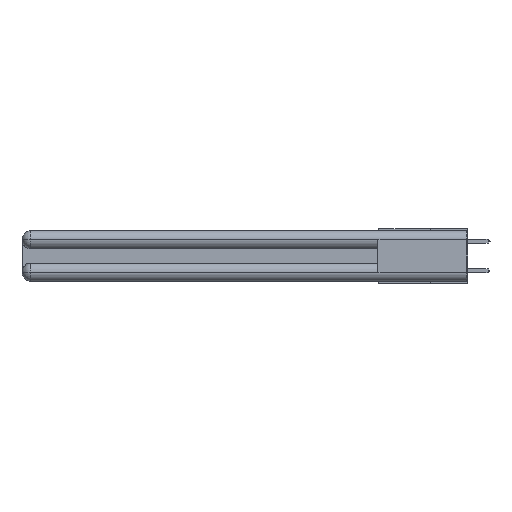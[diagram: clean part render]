
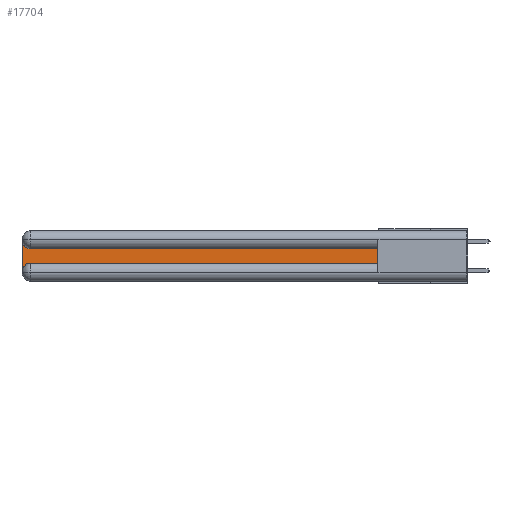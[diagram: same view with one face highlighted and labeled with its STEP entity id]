
A CAD part, left-side view. The second image highlights one B-rep face of the part: STEP entity #17704.
In plain terms, the highlighted planar face has unit normal (-1, 0, 0).
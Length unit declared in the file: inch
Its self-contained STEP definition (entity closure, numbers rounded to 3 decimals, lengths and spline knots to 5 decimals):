
#443 = DIRECTION ( 'NONE',  ( 1., 0., 0. ) ) ;
#962 = EDGE_CURVE ( 'NONE', #9273, #19125, #4611, .T. ) ;
#1816 = CARTESIAN_POINT ( 'NONE',  ( 0.075, 2.94, -0.2175 ) ) ;
#1875 = EDGE_CURVE ( 'NONE', #1937, #10689, #21821, .T. ) ;
#1937 = VERTEX_POINT ( 'NONE', #1816 ) ;
#2377 = VERTEX_POINT ( 'NONE', #25265 ) ;
#2406 = ORIENTED_EDGE ( 'NONE', *, *, #14257, .T. ) ;
#2593 = VECTOR ( 'NONE', #4410, 39.37008 ) ;
#2732 = EDGE_CURVE ( 'NONE', #2377, #9273, #5535, .T. ) ;
#2808 = LINE ( 'NONE', #8001, #10521 ) ;
#3975 = DIRECTION ( 'NONE',  ( 1., 0., 0. ) ) ;
#4410 = DIRECTION ( 'NONE',  ( 0., -1., 0. ) ) ;
#4611 = CIRCLE ( 'NONE', #12810, 0.06 ) ;
#5535 = LINE ( 'NONE', #18310, #6870 ) ;
#5995 = VERTEX_POINT ( 'NONE', #20869 ) ;
#6175 = PLANE ( 'NONE',  #15410 ) ;
#6462 = EDGE_CURVE ( 'NONE', #5995, #1937, #10654, .T. ) ;
#6870 = VECTOR ( 'NONE', #24496, 39.37008 ) ;
#7831 = DIRECTION ( 'NONE',  ( 0., 0., -1. ) ) ;
#8001 = CARTESIAN_POINT ( 'NONE',  ( 0.075, 3., -0.2175 ) ) ;
#8190 = DIRECTION ( 'NONE',  ( 0., 0., -1. ) ) ;
#9062 = ORIENTED_EDGE ( 'NONE', *, *, #962, .T. ) ;
#9273 = VERTEX_POINT ( 'NONE', #27120 ) ;
#10521 = VECTOR ( 'NONE', #7831, 39.37008 ) ;
#10654 = CIRCLE ( 'NONE', #26063, 0.06 ) ;
#10689 = VERTEX_POINT ( 'NONE', #24043 ) ;
#12810 = AXIS2_PLACEMENT_3D ( 'NONE', #13151, #443, #12981 ) ;
#12981 = DIRECTION ( 'NONE',  ( 0., 0., -1. ) ) ;
#13151 = CARTESIAN_POINT ( 'NONE',  ( 0.075, 2.94, -0.0625 ) ) ;
#14144 = FACE_OUTER_BOUND ( 'NONE', #23009, .T. ) ;
#14257 = EDGE_CURVE ( 'NONE', #19125, #5995, #2808, .T. ) ;
#14815 = ORIENTED_EDGE ( 'NONE', *, *, #1875, .T. ) ;
#15082 = CARTESIAN_POINT ( 'NONE',  ( 0.075, 0.6, -0.2175 ) ) ;
#15124 = CARTESIAN_POINT ( 'NONE',  ( 0.075, 0.6, -0.2175 ) ) ;
#15410 = AXIS2_PLACEMENT_3D ( 'NONE', #27057, #16490, #27129 ) ;
#16490 = DIRECTION ( 'NONE',  ( 1., 0., 0. ) ) ;
#16824 = ORIENTED_EDGE ( 'NONE', *, *, #2732, .T. ) ;
#17704 = ADVANCED_FACE ( 'NONE', ( #14144 ), #6175, .F. ) ;
#17823 = ORIENTED_EDGE ( 'NONE', *, *, #27001, .T. ) ;
#18294 = ORIENTED_EDGE ( 'NONE', *, *, #6462, .T. ) ;
#18310 = CARTESIAN_POINT ( 'NONE',  ( 0.075, 0.6, -0.1225 ) ) ;
#18866 = VECTOR ( 'NONE', #19548, 39.37008 ) ;
#19125 = VERTEX_POINT ( 'NONE', #22428 ) ;
#19548 = DIRECTION ( 'NONE',  ( 0., 0., 1. ) ) ;
#20838 = CARTESIAN_POINT ( 'NONE',  ( 0.075, 2.94, -0.2775 ) ) ;
#20869 = CARTESIAN_POINT ( 'NONE',  ( 0.075, 3., -0.2775 ) ) ;
#21821 = LINE ( 'NONE', #15082, #2593 ) ;
#22428 = CARTESIAN_POINT ( 'NONE',  ( 0.075, 3., -0.0625 ) ) ;
#23009 = EDGE_LOOP ( 'NONE', ( #16824, #9062, #2406, #18294, #14815, #17823 ) ) ;
#24043 = CARTESIAN_POINT ( 'NONE',  ( 0.075, 0.6, -0.2175 ) ) ;
#24496 = DIRECTION ( 'NONE',  ( 0., 1., 0. ) ) ;
#25265 = CARTESIAN_POINT ( 'NONE',  ( 0.075, 0.6, -0.1225 ) ) ;
#26063 = AXIS2_PLACEMENT_3D ( 'NONE', #20838, #3975, #8190 ) ;
#27001 = EDGE_CURVE ( 'NONE', #10689, #2377, #27182, .T. ) ;
#27057 = CARTESIAN_POINT ( 'NONE',  ( 0.075, 3., -0.1225 ) ) ;
#27120 = CARTESIAN_POINT ( 'NONE',  ( 0.075, 2.94, -0.1225 ) ) ;
#27129 = DIRECTION ( 'NONE',  ( 0., 0., -1. ) ) ;
#27182 = LINE ( 'NONE', #15124, #18866 ) ;
